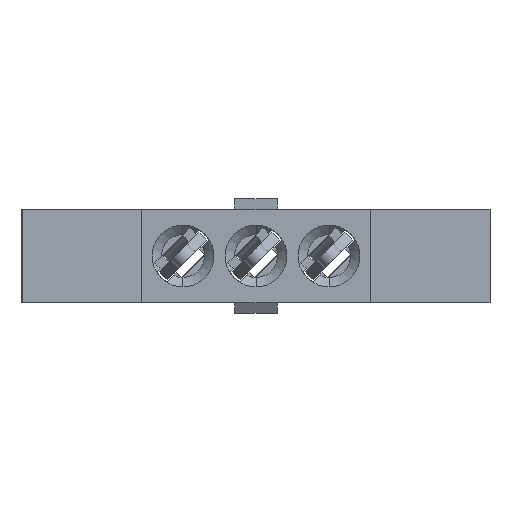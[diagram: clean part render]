
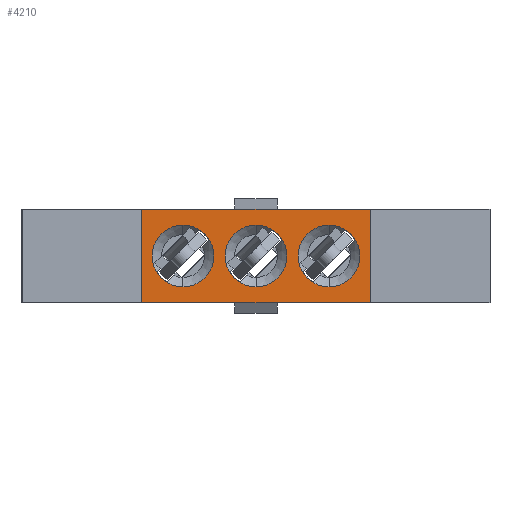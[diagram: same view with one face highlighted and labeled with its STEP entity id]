
A CAD part, front view. The second image highlights one B-rep face of the part: STEP entity #4210.
In plain terms, the highlighted planar face has unit normal (0, -1, 0).
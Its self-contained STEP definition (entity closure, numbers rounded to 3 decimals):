
#61 = CARTESIAN_POINT ( 'NONE',  ( -2.235, -11.176, -2.54 ) ) ;
#126 = ORIENTED_EDGE ( 'NONE', *, *, #2115, .T. ) ;
#159 = CIRCLE ( 'NONE', #3756, 1.676 ) ;
#183 = EDGE_CURVE ( 'NONE', #2021, #3431, #4406, .T. ) ;
#274 = CIRCLE ( 'NONE', #5167, 1.676 ) ;
#452 = FACE_BOUND ( 'NONE', #3314, .T. ) ;
#495 = DIRECTION ( 'NONE',  ( 0., 0., 1. ) ) ;
#574 = CARTESIAN_POINT ( 'NONE',  ( 7.925, -11.176, 0. ) ) ;
#597 = DIRECTION ( 'NONE',  ( 0., 1., 0. ) ) ;
#662 = AXIS2_PLACEMENT_3D ( 'NONE', #574, #597, #4208 ) ;
#817 = ORIENTED_EDGE ( 'NONE', *, *, #2862, .F. ) ;
#846 = CARTESIAN_POINT ( 'NONE',  ( 10.16, -11.176, -2.54 ) ) ;
#916 = CARTESIAN_POINT ( 'NONE',  ( 0., -11.176, 0. ) ) ;
#988 = CARTESIAN_POINT ( 'NONE',  ( 7.925, -11.176, -1.676 ) ) ;
#1023 = FACE_BOUND ( 'NONE', #6373, .T. ) ;
#1170 = ORIENTED_EDGE ( 'NONE', *, *, #3366, .F. ) ;
#1280 = ORIENTED_EDGE ( 'NONE', *, *, #183, .T. ) ;
#1293 = EDGE_LOOP ( 'NONE', ( #1280, #5002 ) ) ;
#1428 = EDGE_LOOP ( 'NONE', ( #5435, #817, #2365, #1170 ) ) ;
#1431 = CIRCLE ( 'NONE', #662, 1.676 ) ;
#1437 = LINE ( 'NONE', #3111, #5165 ) ;
#1551 = CARTESIAN_POINT ( 'NONE',  ( 10.16, -11.176, -2.54 ) ) ;
#1573 = VECTOR ( 'NONE', #4661, 1000. ) ;
#1731 = CARTESIAN_POINT ( 'NONE',  ( 3.962, -11.176, 0. ) ) ;
#1783 = VECTOR ( 'NONE', #4428, 1000. ) ;
#2021 = VERTEX_POINT ( 'NONE', #5075 ) ;
#2115 = EDGE_CURVE ( 'NONE', #5722, #5762, #159, .T. ) ;
#2287 = CIRCLE ( 'NONE', #5006, 1.676 ) ;
#2365 = ORIENTED_EDGE ( 'NONE', *, *, #3286, .F. ) ;
#2401 = CARTESIAN_POINT ( 'NONE',  ( 3.962, -11.176, 0. ) ) ;
#2453 = AXIS2_PLACEMENT_3D ( 'NONE', #916, #3017, #6541 ) ;
#2456 = CARTESIAN_POINT ( 'NONE',  ( 7.925, -11.176, 0. ) ) ;
#2482 = PLANE ( 'NONE',  #2453 ) ;
#2513 = ORIENTED_EDGE ( 'NONE', *, *, #6672, .T. ) ;
#2757 = DIRECTION ( 'NONE',  ( 0., 0., 1. ) ) ;
#2862 = EDGE_CURVE ( 'NONE', #2935, #5191, #4342, .T. ) ;
#2932 = DIRECTION ( 'NONE',  ( 0., 0., 1. ) ) ;
#2935 = VERTEX_POINT ( 'NONE', #1551 ) ;
#3017 = DIRECTION ( 'NONE',  ( 0., 1., 0. ) ) ;
#3030 = VERTEX_POINT ( 'NONE', #6313 ) ;
#3111 = CARTESIAN_POINT ( 'NONE',  ( -2.235, -11.176, 2.54 ) ) ;
#3118 = CARTESIAN_POINT ( 'NONE',  ( -2.235, -11.176, -2.54 ) ) ;
#3185 = ORIENTED_EDGE ( 'NONE', *, *, #5658, .T. ) ;
#3286 = EDGE_CURVE ( 'NONE', #5793, #2935, #3364, .T. ) ;
#3306 = CARTESIAN_POINT ( 'NONE',  ( 0., -11.176, 1.676 ) ) ;
#3314 = EDGE_LOOP ( 'NONE', ( #3185, #126 ) ) ;
#3364 = LINE ( 'NONE', #846, #1783 ) ;
#3366 = EDGE_CURVE ( 'NONE', #3030, #5793, #1437, .T. ) ;
#3427 = ORIENTED_EDGE ( 'NONE', *, *, #4276, .T. ) ;
#3431 = VERTEX_POINT ( 'NONE', #4173 ) ;
#3482 = VERTEX_POINT ( 'NONE', #988 ) ;
#3609 = DIRECTION ( 'NONE',  ( 0., 0., 1. ) ) ;
#3646 = DIRECTION ( 'NONE',  ( 1., 0., 0. ) ) ;
#3682 = CARTESIAN_POINT ( 'NONE',  ( 0., -11.176, -1.676 ) ) ;
#3756 = AXIS2_PLACEMENT_3D ( 'NONE', #5696, #6178, #3609 ) ;
#3795 = VECTOR ( 'NONE', #495, 1000. ) ;
#4173 = CARTESIAN_POINT ( 'NONE',  ( 3.962, -11.176, -1.676 ) ) ;
#4184 = DIRECTION ( 'NONE',  ( 0., 1., 0. ) ) ;
#4208 = DIRECTION ( 'NONE',  ( 0., 0., 1. ) ) ;
#4210 = ADVANCED_FACE ( 'NONE', ( #1023, #4927, #452, #4434 ), #2482, .F. ) ;
#4276 = EDGE_CURVE ( 'NONE', #6448, #3482, #1431, .T. ) ;
#4342 = LINE ( 'NONE', #61, #1573 ) ;
#4363 = DIRECTION ( 'NONE',  ( 0., 1., 0. ) ) ;
#4406 = CIRCLE ( 'NONE', #6328, 1.676 ) ;
#4428 = DIRECTION ( 'NONE',  ( 0., 0., -1. ) ) ;
#4434 = FACE_OUTER_BOUND ( 'NONE', #1428, .T. ) ;
#4639 = CARTESIAN_POINT ( 'NONE',  ( -2.235, -11.176, -2.54 ) ) ;
#4661 = DIRECTION ( 'NONE',  ( -1., 0., 0. ) ) ;
#4927 = FACE_BOUND ( 'NONE', #1293, .T. ) ;
#5002 = ORIENTED_EDGE ( 'NONE', *, *, #5723, .T. ) ;
#5006 = AXIS2_PLACEMENT_3D ( 'NONE', #2456, #6051, #6579 ) ;
#5075 = CARTESIAN_POINT ( 'NONE',  ( 3.962, -11.176, 1.676 ) ) ;
#5135 = LINE ( 'NONE', #3118, #3795 ) ;
#5165 = VECTOR ( 'NONE', #3646, 1000. ) ;
#5167 = AXIS2_PLACEMENT_3D ( 'NONE', #1731, #4363, #2757 ) ;
#5191 = VERTEX_POINT ( 'NONE', #4639 ) ;
#5228 = DIRECTION ( 'NONE',  ( 0., 0., 1. ) ) ;
#5255 = CARTESIAN_POINT ( 'NONE',  ( 0., -11.176, 0. ) ) ;
#5435 = ORIENTED_EDGE ( 'NONE', *, *, #5571, .F. ) ;
#5444 = DIRECTION ( 'NONE',  ( 0., 1., 0. ) ) ;
#5571 = EDGE_CURVE ( 'NONE', #5191, #3030, #5135, .T. ) ;
#5658 = EDGE_CURVE ( 'NONE', #5762, #5722, #6366, .T. ) ;
#5696 = CARTESIAN_POINT ( 'NONE',  ( 0., -11.176, 0. ) ) ;
#5722 = VERTEX_POINT ( 'NONE', #3682 ) ;
#5723 = EDGE_CURVE ( 'NONE', #3431, #2021, #274, .T. ) ;
#5762 = VERTEX_POINT ( 'NONE', #3306 ) ;
#5793 = VERTEX_POINT ( 'NONE', #6526 ) ;
#6051 = DIRECTION ( 'NONE',  ( 0., 1., 0. ) ) ;
#6073 = CARTESIAN_POINT ( 'NONE',  ( 7.925, -11.176, 1.676 ) ) ;
#6178 = DIRECTION ( 'NONE',  ( 0., 1., 0. ) ) ;
#6313 = CARTESIAN_POINT ( 'NONE',  ( -2.235, -11.176, 2.54 ) ) ;
#6328 = AXIS2_PLACEMENT_3D ( 'NONE', #2401, #5444, #2932 ) ;
#6366 = CIRCLE ( 'NONE', #6657, 1.676 ) ;
#6373 = EDGE_LOOP ( 'NONE', ( #3427, #2513 ) ) ;
#6448 = VERTEX_POINT ( 'NONE', #6073 ) ;
#6526 = CARTESIAN_POINT ( 'NONE',  ( 10.16, -11.176, 2.54 ) ) ;
#6541 = DIRECTION ( 'NONE',  ( 0., 0., 1. ) ) ;
#6579 = DIRECTION ( 'NONE',  ( 0., 0., 1. ) ) ;
#6657 = AXIS2_PLACEMENT_3D ( 'NONE', #5255, #4184, #5228 ) ;
#6672 = EDGE_CURVE ( 'NONE', #3482, #6448, #2287, .T. ) ;
